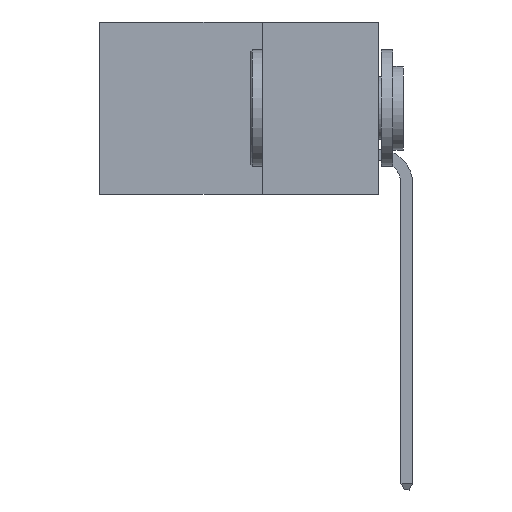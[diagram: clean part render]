
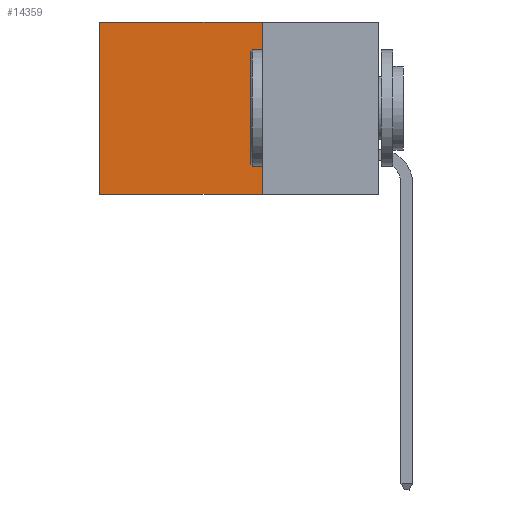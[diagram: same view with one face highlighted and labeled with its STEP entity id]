
A CAD part, left-side view. The second image highlights one B-rep face of the part: STEP entity #14359.
In plain terms, the highlighted planar face has unit normal (-1, 0, 0).
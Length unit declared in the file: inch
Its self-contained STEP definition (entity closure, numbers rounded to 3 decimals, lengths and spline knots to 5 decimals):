
#1235 = EDGE_CURVE ( 'NONE', #13983, #2269, #8447, .T. ) ;
#1485 = VECTOR ( 'NONE', #2446, 39.37008 ) ;
#1588 = FACE_OUTER_BOUND ( 'NONE', #11058, .T. ) ;
#1715 = DIRECTION ( 'NONE',  ( 0., 1., 0. ) ) ;
#2269 = VERTEX_POINT ( 'NONE', #4228 ) ;
#2446 = DIRECTION ( 'NONE',  ( 0., 0., -1. ) ) ;
#2720 = PLANE ( 'NONE',  #6680 ) ;
#2823 = CARTESIAN_POINT ( 'NONE',  ( 0.298, 0.6, 0. ) ) ;
#3759 = VERTEX_POINT ( 'NONE', #8659 ) ;
#3882 = CARTESIAN_POINT ( 'NONE',  ( 0.298, 0.25, 0. ) ) ;
#4228 = CARTESIAN_POINT ( 'NONE',  ( 0.298, 0.6, -0.37 ) ) ;
#4237 = CARTESIAN_POINT ( 'NONE',  ( 0.298, 0.25, -0.37 ) ) ;
#4348 = LINE ( 'NONE', #2823, #7386 ) ;
#4998 = DIRECTION ( 'NONE',  ( 1., 0., 0. ) ) ;
#5755 = EDGE_CURVE ( 'NONE', #3759, #14471, #9617, .T. ) ;
#6478 = VECTOR ( 'NONE', #1715, 39.37008 ) ;
#6544 = ORIENTED_EDGE ( 'NONE', *, *, #9070, .F. ) ;
#6680 = AXIS2_PLACEMENT_3D ( 'NONE', #3882, #4998, #13100 ) ;
#7386 = VECTOR ( 'NONE', #12074, 39.37008 ) ;
#7611 = ORIENTED_EDGE ( 'NONE', *, *, #5755, .T. ) ;
#8062 = VECTOR ( 'NONE', #8588, 39.37008 ) ;
#8447 = LINE ( 'NONE', #8478, #8062 ) ;
#8478 = CARTESIAN_POINT ( 'NONE',  ( 0.298, 0.25, -0.37 ) ) ;
#8588 = DIRECTION ( 'NONE',  ( 0., 1., 0. ) ) ;
#8659 = CARTESIAN_POINT ( 'NONE',  ( 0.298, 0.25, 0. ) ) ;
#8739 = CARTESIAN_POINT ( 'NONE',  ( 0.298, 0.6, 0. ) ) ;
#9070 = EDGE_CURVE ( 'NONE', #3759, #13983, #14015, .T. ) ;
#9342 = EDGE_CURVE ( 'NONE', #14471, #2269, #4348, .T. ) ;
#9617 = LINE ( 'NONE', #9810, #6478 ) ;
#9810 = CARTESIAN_POINT ( 'NONE',  ( 0.298, 0.25, 0. ) ) ;
#10437 = ORIENTED_EDGE ( 'NONE', *, *, #1235, .F. ) ;
#10541 = CARTESIAN_POINT ( 'NONE',  ( 0.298, 0.25, 0. ) ) ;
#11058 = EDGE_LOOP ( 'NONE', ( #11464, #10437, #6544, #7611 ) ) ;
#11464 = ORIENTED_EDGE ( 'NONE', *, *, #9342, .T. ) ;
#12074 = DIRECTION ( 'NONE',  ( 0., 0., -1. ) ) ;
#13100 = DIRECTION ( 'NONE',  ( 0., 0., -1. ) ) ;
#13983 = VERTEX_POINT ( 'NONE', #4237 ) ;
#14015 = LINE ( 'NONE', #10541, #1485 ) ;
#14359 = ADVANCED_FACE ( 'NONE', ( #1588 ), #2720, .F. ) ;
#14471 = VERTEX_POINT ( 'NONE', #8739 ) ;
